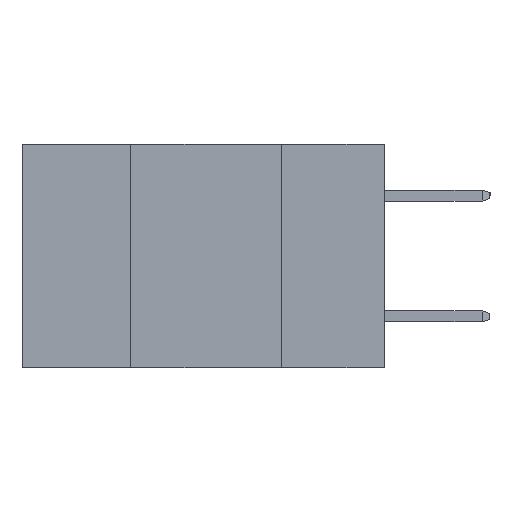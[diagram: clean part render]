
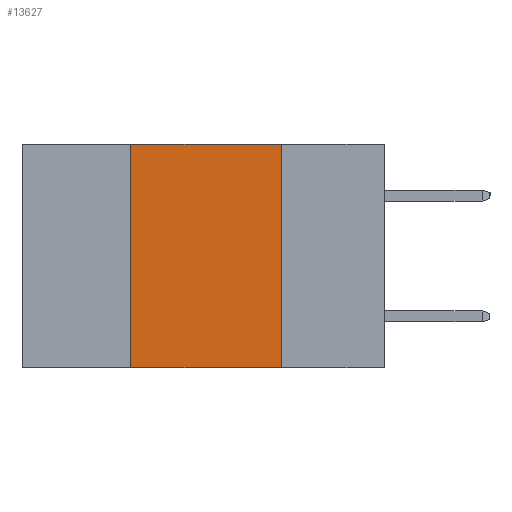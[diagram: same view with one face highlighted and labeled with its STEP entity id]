
A CAD part, left-side view. The second image highlights one B-rep face of the part: STEP entity #13627.
In plain terms, the highlighted planar face has unit normal (-1, 0, 0).
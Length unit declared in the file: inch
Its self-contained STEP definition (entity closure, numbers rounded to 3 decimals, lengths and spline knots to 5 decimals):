
#331 = EDGE_CURVE ( 'NONE', #1322, #5703, #13912, .T. ) ;
#518 = LINE ( 'NONE', #12234, #14474 ) ;
#1317 = EDGE_CURVE ( 'NONE', #1322, #5453, #4357, .T. ) ;
#1322 = VERTEX_POINT ( 'NONE', #13969 ) ;
#1668 = VECTOR ( 'NONE', #13621, 39.37008 ) ;
#2302 = DIRECTION ( 'NONE',  ( 0., 0., -1. ) ) ;
#2351 = DIRECTION ( 'NONE',  ( 0., 0., 1. ) ) ;
#2745 = ORIENTED_EDGE ( 'NONE', *, *, #1317, .T. ) ;
#3792 = CARTESIAN_POINT ( 'NONE',  ( 0., 0.42, 0. ) ) ;
#4357 = LINE ( 'NONE', #8943, #1668 ) ;
#4406 = AXIS2_PLACEMENT_3D ( 'NONE', #4613, #5578, #2302 ) ;
#4457 = CARTESIAN_POINT ( 'NONE',  ( 0., 0.17, 0. ) ) ;
#4613 = CARTESIAN_POINT ( 'NONE',  ( 0., 0.6, 0. ) ) ;
#5276 = VECTOR ( 'NONE', #7020, 39.37008 ) ;
#5453 = VERTEX_POINT ( 'NONE', #8526 ) ;
#5578 = DIRECTION ( 'NONE',  ( 1., 0., 0. ) ) ;
#5703 = VERTEX_POINT ( 'NONE', #3792 ) ;
#5725 = PLANE ( 'NONE',  #4406 ) ;
#5795 = ORIENTED_EDGE ( 'NONE', *, *, #331, .F. ) ;
#6115 = VECTOR ( 'NONE', #2351, 39.37008 ) ;
#6142 = LINE ( 'NONE', #11721, #5276 ) ;
#6267 = EDGE_LOOP ( 'NONE', ( #8024, #14646, #5795, #2745 ) ) ;
#7020 = DIRECTION ( 'NONE',  ( 0., 0., -1. ) ) ;
#7280 = VERTEX_POINT ( 'NONE', #4457 ) ;
#8024 = ORIENTED_EDGE ( 'NONE', *, *, #8553, .F. ) ;
#8526 = CARTESIAN_POINT ( 'NONE',  ( 0., 0.17, -0.37 ) ) ;
#8553 = EDGE_CURVE ( 'NONE', #7280, #5453, #6142, .T. ) ;
#8943 = CARTESIAN_POINT ( 'NONE',  ( 0., 0.6, -0.37 ) ) ;
#11114 = DIRECTION ( 'NONE',  ( 0., -1., 0. ) ) ;
#11721 = CARTESIAN_POINT ( 'NONE',  ( 0., 0.17, -0.37 ) ) ;
#11838 = EDGE_CURVE ( 'NONE', #5703, #7280, #518, .T. ) ;
#12234 = CARTESIAN_POINT ( 'NONE',  ( 0., 0.6, 0. ) ) ;
#12711 = CARTESIAN_POINT ( 'NONE',  ( 0., 0.42, -0.37 ) ) ;
#13621 = DIRECTION ( 'NONE',  ( 0., -1., 0. ) ) ;
#13627 = ADVANCED_FACE ( 'NONE', ( #14870 ), #5725, .F. ) ;
#13912 = LINE ( 'NONE', #12711, #6115 ) ;
#13969 = CARTESIAN_POINT ( 'NONE',  ( 0., 0.42, -0.37 ) ) ;
#14474 = VECTOR ( 'NONE', #11114, 39.37008 ) ;
#14646 = ORIENTED_EDGE ( 'NONE', *, *, #11838, .F. ) ;
#14870 = FACE_OUTER_BOUND ( 'NONE', #6267, .T. ) ;
